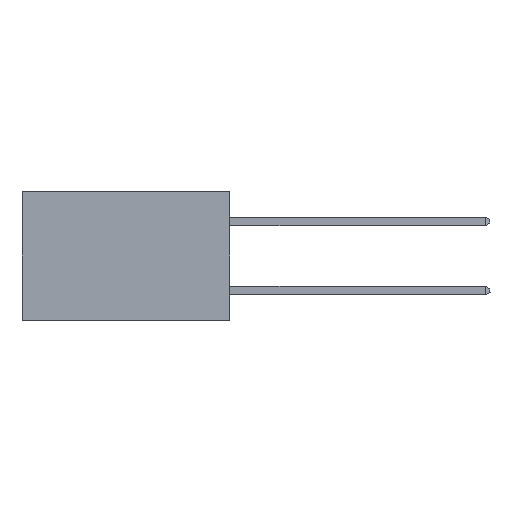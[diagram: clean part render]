
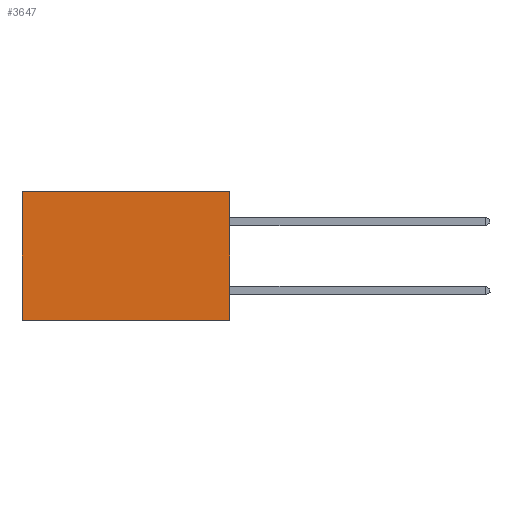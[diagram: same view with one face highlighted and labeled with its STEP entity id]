
A CAD part, left-side view. The second image highlights one B-rep face of the part: STEP entity #3647.
In plain terms, the highlighted planar face has unit normal (-1, 0, 0).
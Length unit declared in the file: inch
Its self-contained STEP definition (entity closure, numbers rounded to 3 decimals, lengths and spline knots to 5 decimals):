
#518 = ORIENTED_EDGE ( 'NONE', *, *, #13716, .F. ) ;
#615 = VERTEX_POINT ( 'NONE', #10584 ) ;
#1128 = VERTEX_POINT ( 'NONE', #30442 ) ;
#1425 = VECTOR ( 'NONE', #9201, 39.37008 ) ;
#2038 = DIRECTION ( 'NONE',  ( 0., 0., -1. ) ) ;
#2157 = ORIENTED_EDGE ( 'NONE', *, *, #19194, .F. ) ;
#2592 = CARTESIAN_POINT ( 'NONE',  ( 0.298, 0., 0. ) ) ;
#3033 = CARTESIAN_POINT ( 'NONE',  ( 0.298, 0., 0. ) ) ;
#3647 = ADVANCED_FACE ( 'NONE', ( #18999 ), #19135, .F. ) ;
#4380 = CARTESIAN_POINT ( 'NONE',  ( 0.298, 0., -0.37 ) ) ;
#5686 = EDGE_LOOP ( 'NONE', ( #23984, #2157, #518, #17257 ) ) ;
#7016 = DIRECTION ( 'NONE',  ( 1., 0., 0. ) ) ;
#7226 = CARTESIAN_POINT ( 'NONE',  ( 0.298, 0., -0.37 ) ) ;
#9201 = DIRECTION ( 'NONE',  ( 0., 1., 0. ) ) ;
#10584 = CARTESIAN_POINT ( 'NONE',  ( 0.298, 0.6, -0.37 ) ) ;
#11584 = AXIS2_PLACEMENT_3D ( 'NONE', #11870, #7016, #2038 ) ;
#11870 = CARTESIAN_POINT ( 'NONE',  ( 0.298, 0., 0. ) ) ;
#12508 = CARTESIAN_POINT ( 'NONE',  ( 0.298, 0., 0. ) ) ;
#12681 = DIRECTION ( 'NONE',  ( 0., 0., -1. ) ) ;
#12863 = VERTEX_POINT ( 'NONE', #7226 ) ;
#12881 = VECTOR ( 'NONE', #12681, 39.37008 ) ;
#12956 = VERTEX_POINT ( 'NONE', #12508 ) ;
#13716 = EDGE_CURVE ( 'NONE', #12956, #12863, #25652, .T. ) ;
#14345 = LINE ( 'NONE', #4380, #1425 ) ;
#17127 = DIRECTION ( 'NONE',  ( 0., 1., 0. ) ) ;
#17257 = ORIENTED_EDGE ( 'NONE', *, *, #29865, .T. ) ;
#18064 = CARTESIAN_POINT ( 'NONE',  ( 0.298, 0.6, 0. ) ) ;
#18999 = FACE_OUTER_BOUND ( 'NONE', #5686, .T. ) ;
#19135 = PLANE ( 'NONE',  #11584 ) ;
#19194 = EDGE_CURVE ( 'NONE', #12863, #615, #14345, .T. ) ;
#22027 = LINE ( 'NONE', #2592, #26947 ) ;
#23984 = ORIENTED_EDGE ( 'NONE', *, *, #28190, .T. ) ;
#24038 = VECTOR ( 'NONE', #25389, 39.37008 ) ;
#25389 = DIRECTION ( 'NONE',  ( 0., 0., -1. ) ) ;
#25652 = LINE ( 'NONE', #3033, #12881 ) ;
#26297 = LINE ( 'NONE', #18064, #24038 ) ;
#26947 = VECTOR ( 'NONE', #17127, 39.37008 ) ;
#28190 = EDGE_CURVE ( 'NONE', #1128, #615, #26297, .T. ) ;
#29865 = EDGE_CURVE ( 'NONE', #12956, #1128, #22027, .T. ) ;
#30442 = CARTESIAN_POINT ( 'NONE',  ( 0.298, 0.6, 0. ) ) ;
